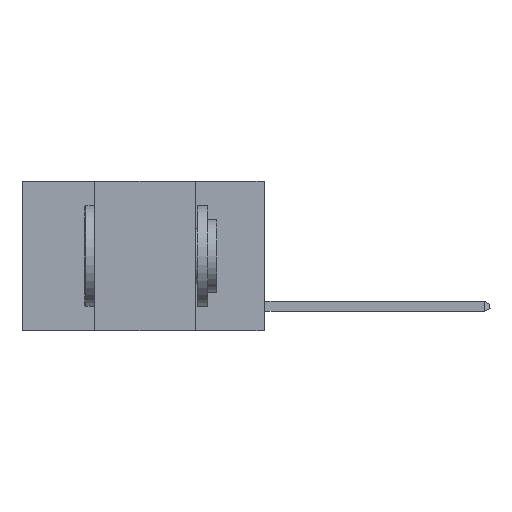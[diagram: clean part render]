
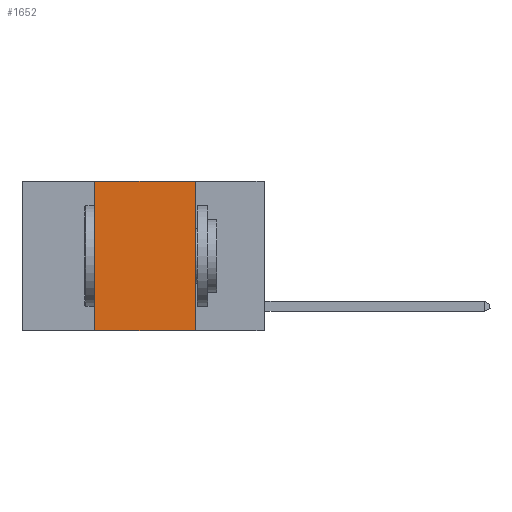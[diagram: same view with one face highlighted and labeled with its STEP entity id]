
A CAD part, left-side view. The second image highlights one B-rep face of the part: STEP entity #1652.
In plain terms, the highlighted planar face has unit normal (-1, 0, 0).
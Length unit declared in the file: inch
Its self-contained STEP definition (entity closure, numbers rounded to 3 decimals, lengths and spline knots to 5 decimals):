
#9 = VECTOR ( 'NONE', #10561, 39.37008 ) ;
#544 = VERTEX_POINT ( 'NONE', #1719 ) ;
#1592 = EDGE_CURVE ( 'NONE', #4990, #544, #8285, .T. ) ;
#1652 = ADVANCED_FACE ( 'NONE', ( #4360 ), #10002, .F. ) ;
#1699 = DIRECTION ( 'NONE',  ( 0., 0., -1. ) ) ;
#1719 = CARTESIAN_POINT ( 'NONE',  ( 0., 0.17, 0. ) ) ;
#2005 = EDGE_LOOP ( 'NONE', ( #10272, #10386, #3406, #5292 ) ) ;
#2036 = VERTEX_POINT ( 'NONE', #3971 ) ;
#3406 = ORIENTED_EDGE ( 'NONE', *, *, #10170, .F. ) ;
#3478 = AXIS2_PLACEMENT_3D ( 'NONE', #9212, #3606, #6939 ) ;
#3606 = DIRECTION ( 'NONE',  ( 1., 0., 0. ) ) ;
#3971 = CARTESIAN_POINT ( 'NONE',  ( 0., 0.42, -0.37 ) ) ;
#4360 = FACE_OUTER_BOUND ( 'NONE', #2005, .T. ) ;
#4990 = VERTEX_POINT ( 'NONE', #6655 ) ;
#5292 = ORIENTED_EDGE ( 'NONE', *, *, #9308, .T. ) ;
#5463 = VERTEX_POINT ( 'NONE', #6164 ) ;
#5564 = CARTESIAN_POINT ( 'NONE',  ( 0., 0.6, -0.37 ) ) ;
#5826 = CARTESIAN_POINT ( 'NONE',  ( 0., 0.17, 0. ) ) ;
#5908 = EDGE_CURVE ( 'NONE', #544, #5463, #6545, .T. ) ;
#6164 = CARTESIAN_POINT ( 'NONE',  ( 0., 0.17, -0.37 ) ) ;
#6393 = VECTOR ( 'NONE', #9461, 39.37008 ) ;
#6545 = LINE ( 'NONE', #5826, #10660 ) ;
#6655 = CARTESIAN_POINT ( 'NONE',  ( 0., 0.42, 0. ) ) ;
#6939 = DIRECTION ( 'NONE',  ( 0., 0., -1. ) ) ;
#7133 = VECTOR ( 'NONE', #8920, 39.37008 ) ;
#7646 = LINE ( 'NONE', #8481, #6393 ) ;
#8285 = LINE ( 'NONE', #10675, #9 ) ;
#8481 = CARTESIAN_POINT ( 'NONE',  ( 0., 0.42, 0. ) ) ;
#8920 = DIRECTION ( 'NONE',  ( 0., -1., 0. ) ) ;
#9212 = CARTESIAN_POINT ( 'NONE',  ( 0., 0.6, 0. ) ) ;
#9308 = EDGE_CURVE ( 'NONE', #2036, #5463, #9725, .T. ) ;
#9461 = DIRECTION ( 'NONE',  ( 0., 0., 1. ) ) ;
#9725 = LINE ( 'NONE', #5564, #7133 ) ;
#10002 = PLANE ( 'NONE',  #3478 ) ;
#10170 = EDGE_CURVE ( 'NONE', #2036, #4990, #7646, .T. ) ;
#10272 = ORIENTED_EDGE ( 'NONE', *, *, #5908, .F. ) ;
#10386 = ORIENTED_EDGE ( 'NONE', *, *, #1592, .F. ) ;
#10561 = DIRECTION ( 'NONE',  ( 0., -1., 0. ) ) ;
#10660 = VECTOR ( 'NONE', #1699, 39.37008 ) ;
#10675 = CARTESIAN_POINT ( 'NONE',  ( 0., 0.6, 0. ) ) ;
